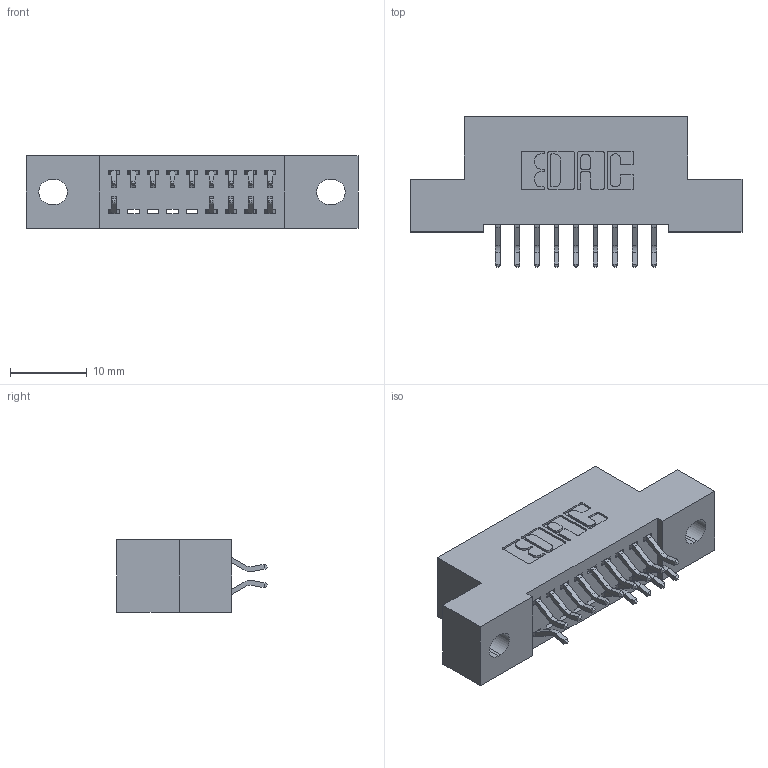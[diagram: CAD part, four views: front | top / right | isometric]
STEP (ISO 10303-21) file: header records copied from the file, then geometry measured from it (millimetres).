
FILE_DESCRIPTION (( 'STEP AP203' ), '1' );
FILE_NAME ('392-018-556-202.STEP', '2018-08-15T04:40:22', ( '' ), ( '' ), 'SwSTEP 2.0', 'SolidWorks 2016', '' );
FILE_SCHEMA (( 'CONFIG_CONTROL_DESIGN' ));
Length unit declared in the file: inch
Products named in the file (3): 392-018-556-202; 342 Part_.128 Slot; 345-292-001_556 Tail
Assembly tree (15 placements, depth 2):
  392-018-556-202
    342 Part_.128 Slot
    345-292-001_556 Tail  x14
Bounding box: 43.18 x 19.58 x 9.4 mm (x, y, z)
Volume: 3635 mm3; surface area: 4650.7 mm2
Topology: 15 solids, 15 shells, 950 faces, 2817 edges, 1858 vertices
Faces by surface type: plane 654, cylinder 296
Entity records: 10153 total; most frequent: CARTESIAN_POINT 1754, ORIENTED_EDGE 1682, DIRECTION 1541, EDGE_CURVE 841, LINE 705, VECTOR 705, VERTEX_POINT 558, AXIS2_PLACEMENT_3D 418
